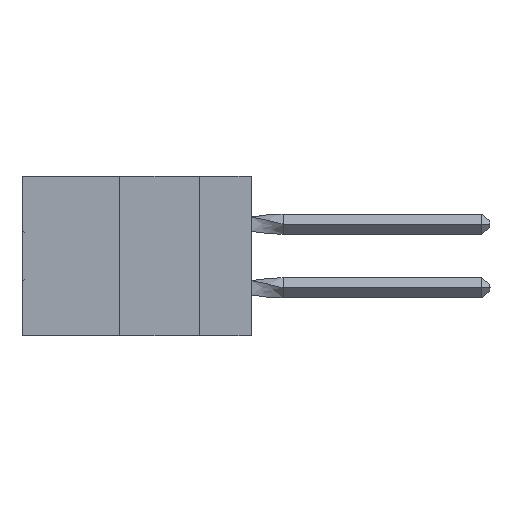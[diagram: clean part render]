
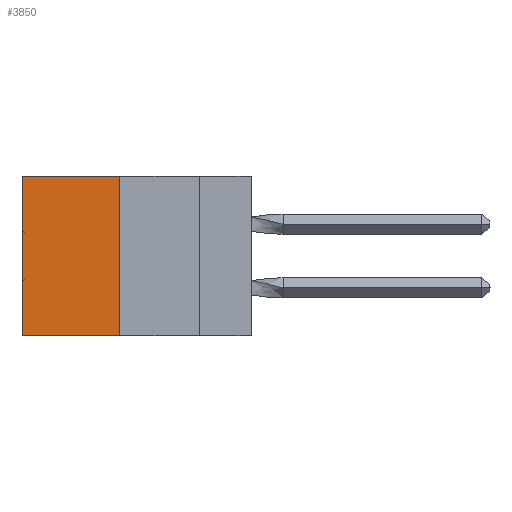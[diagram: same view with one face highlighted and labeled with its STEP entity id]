
A CAD part, left-side view. The second image highlights one B-rep face of the part: STEP entity #3850.
In plain terms, the highlighted planar face has unit normal (-1, 0, 0).
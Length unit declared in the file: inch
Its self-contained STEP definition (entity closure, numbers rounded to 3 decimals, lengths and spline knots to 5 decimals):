
#323 = CARTESIAN_POINT ( 'NONE',  ( 0.305, 0.413, 0. ) ) ;
#2210 = VERTEX_POINT ( 'NONE', #3093 ) ;
#2377 = VECTOR ( 'NONE', #6142, 39.37008 ) ;
#2899 = EDGE_CURVE ( 'NONE', #2210, #51129, #37513, .T. ) ;
#2920 = DIRECTION ( 'NONE',  ( 0., 0., -1. ) ) ;
#3093 = CARTESIAN_POINT ( 'NONE',  ( 0.305, 0.72, 0. ) ) ;
#3850 = ADVANCED_FACE ( 'NONE', ( #17624 ), #19773, .F. ) ;
#6142 = DIRECTION ( 'NONE',  ( 0., 1., 0. ) ) ;
#7879 = CARTESIAN_POINT ( 'NONE',  ( 0.305, 0.72, -0.5 ) ) ;
#8148 = LINE ( 'NONE', #14127, #2377 ) ;
#9035 = EDGE_LOOP ( 'NONE', ( #15846, #12414, #13668, #34560 ) ) ;
#11019 = CARTESIAN_POINT ( 'NONE',  ( 0.305, 0.413, -0.5 ) ) ;
#11602 = DIRECTION ( 'NONE',  ( 0., 0., -1. ) ) ;
#12414 = ORIENTED_EDGE ( 'NONE', *, *, #48442, .F. ) ;
#12964 = AXIS2_PLACEMENT_3D ( 'NONE', #23529, #31509, #11602 ) ;
#13668 = ORIENTED_EDGE ( 'NONE', *, *, #26578, .F. ) ;
#14127 = CARTESIAN_POINT ( 'NONE',  ( 0.305, 0.413, -0.5 ) ) ;
#15846 = ORIENTED_EDGE ( 'NONE', *, *, #2899, .T. ) ;
#17619 = DIRECTION ( 'NONE',  ( 0., 0., -1. ) ) ;
#17624 = FACE_OUTER_BOUND ( 'NONE', #9035, .T. ) ;
#19773 = PLANE ( 'NONE',  #12964 ) ;
#23529 = CARTESIAN_POINT ( 'NONE',  ( 0.305, 0.413, -0.5 ) ) ;
#26578 = EDGE_CURVE ( 'NONE', #31834, #43661, #34420, .T. ) ;
#29549 = VECTOR ( 'NONE', #41641, 39.37008 ) ;
#30526 = VECTOR ( 'NONE', #2920, 39.37008 ) ;
#31509 = DIRECTION ( 'NONE',  ( 1., 0., 0. ) ) ;
#31732 = VECTOR ( 'NONE', #17619, 39.37008 ) ;
#31834 = VERTEX_POINT ( 'NONE', #323 ) ;
#33849 = CARTESIAN_POINT ( 'NONE',  ( 0.305, 0.72, -0.5 ) ) ;
#34420 = LINE ( 'NONE', #47341, #30526 ) ;
#34560 = ORIENTED_EDGE ( 'NONE', *, *, #51939, .T. ) ;
#37513 = LINE ( 'NONE', #33849, #31732 ) ;
#41641 = DIRECTION ( 'NONE',  ( 0., 1., 0. ) ) ;
#43661 = VERTEX_POINT ( 'NONE', #11019 ) ;
#45385 = CARTESIAN_POINT ( 'NONE',  ( 0.305, 0.413, 0. ) ) ;
#47341 = CARTESIAN_POINT ( 'NONE',  ( 0.305, 0.413, -0.5 ) ) ;
#48442 = EDGE_CURVE ( 'NONE', #43661, #51129, #8148, .T. ) ;
#49376 = LINE ( 'NONE', #45385, #29549 ) ;
#51129 = VERTEX_POINT ( 'NONE', #7879 ) ;
#51939 = EDGE_CURVE ( 'NONE', #31834, #2210, #49376, .T. ) ;
